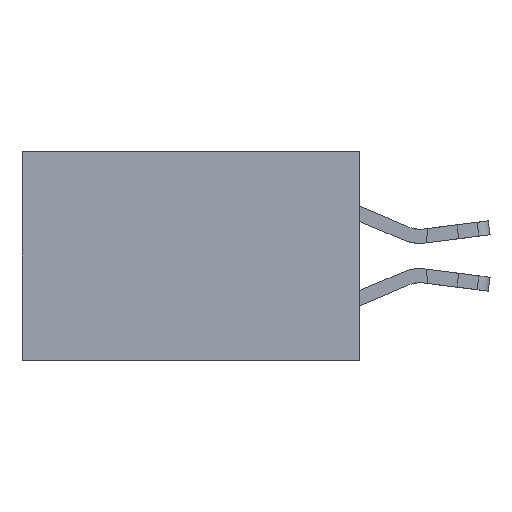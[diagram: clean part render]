
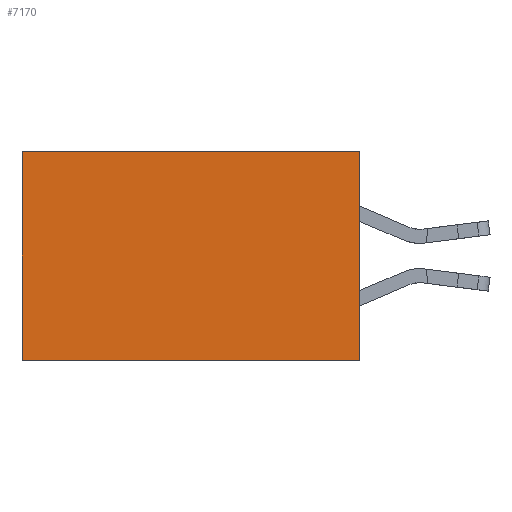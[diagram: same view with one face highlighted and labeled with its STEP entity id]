
A CAD part, left-side view. The second image highlights one B-rep face of the part: STEP entity #7170.
In plain terms, the highlighted planar face has unit normal (-1, 0, 0).
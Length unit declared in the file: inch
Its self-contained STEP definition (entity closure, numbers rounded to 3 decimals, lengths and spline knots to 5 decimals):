
#408 = EDGE_CURVE ( 'NONE', #32926, #5387, #4364, .T. ) ;
#834 = VERTEX_POINT ( 'NONE', #26956 ) ;
#1443 = CARTESIAN_POINT ( 'NONE',  ( 0.2875, 0.6, -0.37 ) ) ;
#3044 = DIRECTION ( 'NONE',  ( 0., 1., 0. ) ) ;
#3911 = CARTESIAN_POINT ( 'NONE',  ( 0.2875, 0., -0.37 ) ) ;
#3912 = PLANE ( 'NONE',  #20551 ) ;
#3913 = VECTOR ( 'NONE', #26486, 39.37008 ) ;
#4364 = LINE ( 'NONE', #9909, #31202 ) ;
#4677 = LINE ( 'NONE', #9607, #9129 ) ;
#5387 = VERTEX_POINT ( 'NONE', #1443 ) ;
#7170 = ADVANCED_FACE ( 'NONE', ( #17252 ), #3912, .F. ) ;
#8510 = EDGE_CURVE ( 'NONE', #11311, #5387, #29363, .T. ) ;
#8999 = EDGE_LOOP ( 'NONE', ( #16983, #24386, #31750, #32201 ) ) ;
#9129 = VECTOR ( 'NONE', #9383, 39.37008 ) ;
#9383 = DIRECTION ( 'NONE',  ( 0., 1., 0. ) ) ;
#9607 = CARTESIAN_POINT ( 'NONE',  ( 0.2875, 0., 0. ) ) ;
#9909 = CARTESIAN_POINT ( 'NONE',  ( 0.2875, 0.6, 0. ) ) ;
#10830 = LINE ( 'NONE', #18302, #3913 ) ;
#11067 = VECTOR ( 'NONE', #3044, 39.37008 ) ;
#11311 = VERTEX_POINT ( 'NONE', #32485 ) ;
#13677 = EDGE_CURVE ( 'NONE', #834, #32926, #4677, .T. ) ;
#14274 = DIRECTION ( 'NONE',  ( 0., 0., -1. ) ) ;
#16983 = ORIENTED_EDGE ( 'NONE', *, *, #408, .T. ) ;
#17252 = FACE_OUTER_BOUND ( 'NONE', #8999, .T. ) ;
#18302 = CARTESIAN_POINT ( 'NONE',  ( 0.2875, 0., 0. ) ) ;
#19271 = CARTESIAN_POINT ( 'NONE',  ( 0.2875, 0., 0. ) ) ;
#19785 = CARTESIAN_POINT ( 'NONE',  ( 0.2875, 0.6, 0. ) ) ;
#20551 = AXIS2_PLACEMENT_3D ( 'NONE', #19271, #29944, #14274 ) ;
#22994 = DIRECTION ( 'NONE',  ( 0., 0., -1. ) ) ;
#24386 = ORIENTED_EDGE ( 'NONE', *, *, #8510, .F. ) ;
#26486 = DIRECTION ( 'NONE',  ( 0., 0., -1. ) ) ;
#26956 = CARTESIAN_POINT ( 'NONE',  ( 0.2875, 0., 0. ) ) ;
#28799 = EDGE_CURVE ( 'NONE', #834, #11311, #10830, .T. ) ;
#29363 = LINE ( 'NONE', #3911, #11067 ) ;
#29944 = DIRECTION ( 'NONE',  ( 1., 0., 0. ) ) ;
#31202 = VECTOR ( 'NONE', #22994, 39.37008 ) ;
#31750 = ORIENTED_EDGE ( 'NONE', *, *, #28799, .F. ) ;
#32201 = ORIENTED_EDGE ( 'NONE', *, *, #13677, .T. ) ;
#32485 = CARTESIAN_POINT ( 'NONE',  ( 0.2875, 0., -0.37 ) ) ;
#32926 = VERTEX_POINT ( 'NONE', #19785 ) ;
